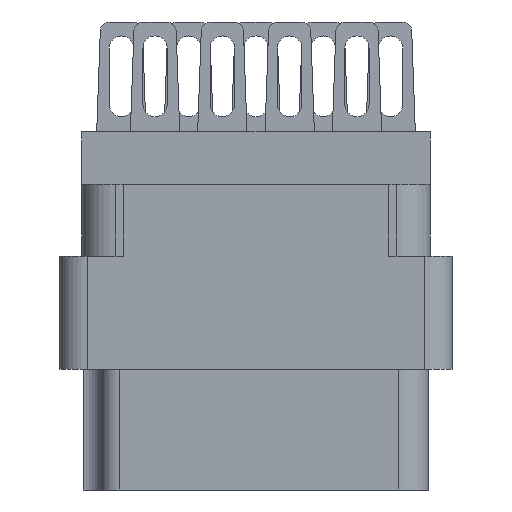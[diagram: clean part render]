
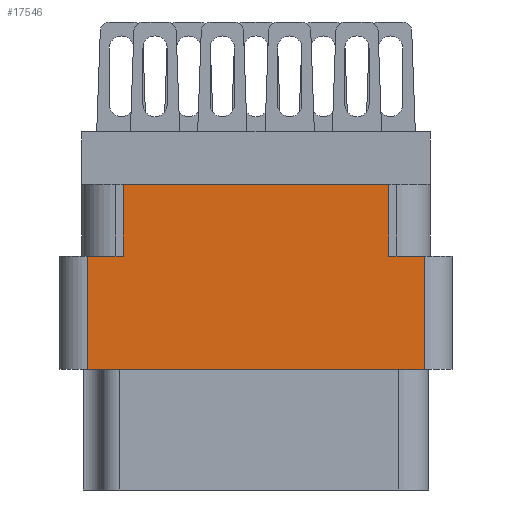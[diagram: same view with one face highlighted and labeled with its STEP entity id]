
A CAD part, left-side view. The second image highlights one B-rep face of the part: STEP entity #17546.
In plain terms, the highlighted planar face has unit normal (-1, 0, 0).
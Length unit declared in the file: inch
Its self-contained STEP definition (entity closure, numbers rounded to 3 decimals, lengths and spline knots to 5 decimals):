
#972 = ORIENTED_EDGE ( 'NONE', *, *, #37890, .F. ) ;
#1057 = DIRECTION ( 'NONE',  ( -1., 0., 0. ) ) ;
#2147 = CARTESIAN_POINT ( 'NONE',  ( -1., 0., -0.529 ) ) ;
#2367 = VECTOR ( 'NONE', #15865, 39.37008 ) ;
#2944 = VERTEX_POINT ( 'NONE', #13692 ) ;
#3182 = DIRECTION ( 'NONE',  ( 0., -1., 0. ) ) ;
#3651 = VECTOR ( 'NONE', #3182, 39.37008 ) ;
#4845 = DIRECTION ( 'NONE',  ( 0., -1., 0. ) ) ;
#5245 = ORIENTED_EDGE ( 'NONE', *, *, #21033, .F. ) ;
#5539 = VECTOR ( 'NONE', #35848, 39.37008 ) ;
#5801 = CARTESIAN_POINT ( 'NONE',  ( -1., 0., -0.277 ) ) ;
#6085 = VECTOR ( 'NONE', #27037, 39.37008 ) ;
#9441 = VERTEX_POINT ( 'NONE', #36246 ) ;
#10165 = FACE_OUTER_BOUND ( 'NONE', #19134, .T. ) ;
#12081 = CARTESIAN_POINT ( 'NONE',  ( -1., -0.296, -0.277 ) ) ;
#12571 = LINE ( 'NONE', #5801, #3651 ) ;
#12767 = CARTESIAN_POINT ( 'NONE',  ( -1., 0.376, -0.529 ) ) ;
#13692 = CARTESIAN_POINT ( 'NONE',  ( -1., -0.376, -0.277 ) ) ;
#13723 = ORIENTED_EDGE ( 'NONE', *, *, #13729, .T. ) ;
#13729 = EDGE_CURVE ( 'NONE', #17623, #20994, #15501, .T. ) ;
#14474 = ORIENTED_EDGE ( 'NONE', *, *, #20409, .T. ) ;
#14552 = LINE ( 'NONE', #15937, #31941 ) ;
#15049 = CARTESIAN_POINT ( 'NONE',  ( -1., 0.296, -0.277 ) ) ;
#15501 = LINE ( 'NONE', #33363, #6085 ) ;
#15865 = DIRECTION ( 'NONE',  ( 0., 0., 1. ) ) ;
#15937 = CARTESIAN_POINT ( 'NONE',  ( -1., 0.438, -0.117 ) ) ;
#16040 = VECTOR ( 'NONE', #36320, 39.37008 ) ;
#16290 = CARTESIAN_POINT ( 'NONE',  ( -1., -0.376, -0.529 ) ) ;
#16512 = ORIENTED_EDGE ( 'NONE', *, *, #21920, .F. ) ;
#16939 = CARTESIAN_POINT ( 'NONE',  ( -1., 0., -0.277 ) ) ;
#17546 = ADVANCED_FACE ( 'NONE', ( #10165 ), #19086, .T. ) ;
#17623 = VERTEX_POINT ( 'NONE', #34167 ) ;
#19086 = PLANE ( 'NONE',  #23955 ) ;
#19134 = EDGE_LOOP ( 'NONE', ( #16512, #13723, #30254, #14474, #972, #28338, #5245, #26249 ) ) ;
#19667 = EDGE_CURVE ( 'NONE', #34485, #9441, #32036, .T. ) ;
#19983 = VECTOR ( 'NONE', #4845, 39.37008 ) ;
#20409 = EDGE_CURVE ( 'NONE', #37781, #2944, #24461, .T. ) ;
#20994 = VERTEX_POINT ( 'NONE', #12767 ) ;
#21033 = EDGE_CURVE ( 'NONE', #9441, #36114, #14552, .T. ) ;
#21920 = EDGE_CURVE ( 'NONE', #17623, #34485, #12571, .T. ) ;
#22515 = VECTOR ( 'NONE', #26195, 39.37008 ) ;
#23955 = AXIS2_PLACEMENT_3D ( 'NONE', #27832, #1057, #36934 ) ;
#24461 = LINE ( 'NONE', #28172, #2367 ) ;
#24535 = EDGE_CURVE ( 'NONE', #36864, #36114, #24790, .T. ) ;
#24790 = LINE ( 'NONE', #12081, #5539 ) ;
#26195 = DIRECTION ( 'NONE',  ( 0., 1., 0. ) ) ;
#26249 = ORIENTED_EDGE ( 'NONE', *, *, #19667, .F. ) ;
#26469 = CARTESIAN_POINT ( 'NONE',  ( -1., -0.296, -0.277 ) ) ;
#27037 = DIRECTION ( 'NONE',  ( 0., 0., -1. ) ) ;
#27832 = CARTESIAN_POINT ( 'NONE',  ( -1., -0.438, -0.798 ) ) ;
#28172 = CARTESIAN_POINT ( 'NONE',  ( -1., -0.376, -0.798 ) ) ;
#28338 = ORIENTED_EDGE ( 'NONE', *, *, #24535, .T. ) ;
#30254 = ORIENTED_EDGE ( 'NONE', *, *, #30663, .F. ) ;
#30663 = EDGE_CURVE ( 'NONE', #37781, #20994, #38498, .T. ) ;
#31788 = CARTESIAN_POINT ( 'NONE',  ( -1., -0.296, -0.117 ) ) ;
#31941 = VECTOR ( 'NONE', #36973, 39.37008 ) ;
#32036 = LINE ( 'NONE', #15049, #16040 ) ;
#32568 = CARTESIAN_POINT ( 'NONE',  ( -1., 0.296, -0.277 ) ) ;
#33363 = CARTESIAN_POINT ( 'NONE',  ( -1., 0.376, -0.798 ) ) ;
#34167 = CARTESIAN_POINT ( 'NONE',  ( -1., 0.376, -0.277 ) ) ;
#34485 = VERTEX_POINT ( 'NONE', #32568 ) ;
#35848 = DIRECTION ( 'NONE',  ( 0., 0., 1. ) ) ;
#35971 = LINE ( 'NONE', #16939, #19983 ) ;
#36114 = VERTEX_POINT ( 'NONE', #31788 ) ;
#36246 = CARTESIAN_POINT ( 'NONE',  ( -1., 0.296, -0.117 ) ) ;
#36320 = DIRECTION ( 'NONE',  ( 0., 0., 1. ) ) ;
#36864 = VERTEX_POINT ( 'NONE', #26469 ) ;
#36934 = DIRECTION ( 'NONE',  ( 0., 0., 1. ) ) ;
#36973 = DIRECTION ( 'NONE',  ( 0., -1., 0. ) ) ;
#37781 = VERTEX_POINT ( 'NONE', #16290 ) ;
#37890 = EDGE_CURVE ( 'NONE', #36864, #2944, #35971, .T. ) ;
#38498 = LINE ( 'NONE', #2147, #22515 ) ;
